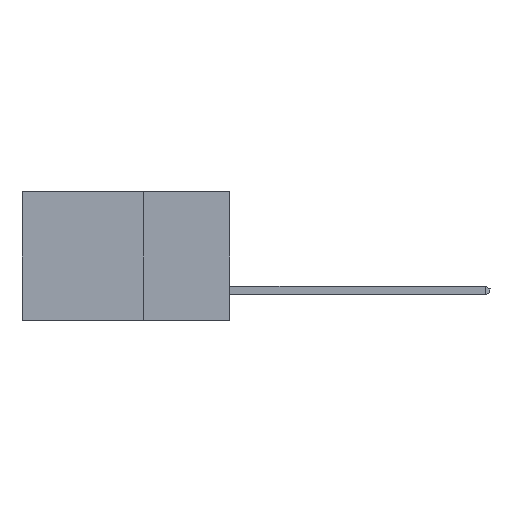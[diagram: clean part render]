
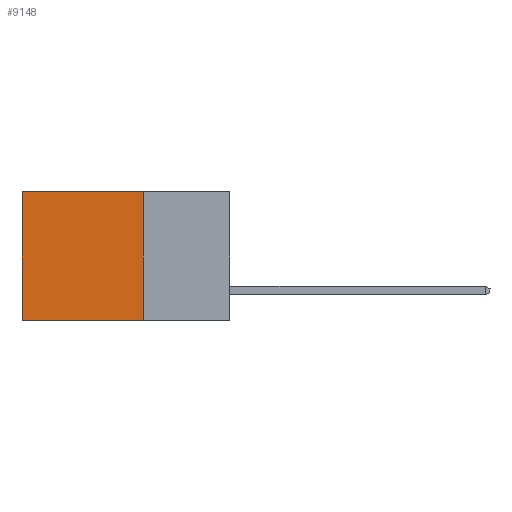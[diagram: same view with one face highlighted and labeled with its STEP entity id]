
A CAD part, left-side view. The second image highlights one B-rep face of the part: STEP entity #9148.
In plain terms, the highlighted planar face has unit normal (-1, 0, 0).
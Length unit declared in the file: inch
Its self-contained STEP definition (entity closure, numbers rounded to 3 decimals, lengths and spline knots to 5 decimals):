
#234 = LINE ( 'NONE', #9749, #6806 ) ;
#680 = ORIENTED_EDGE ( 'NONE', *, *, #12096, .T. ) ;
#724 = LINE ( 'NONE', #6959, #6008 ) ;
#1845 = EDGE_LOOP ( 'NONE', ( #680, #12845, #9667, #8556 ) ) ;
#3047 = VERTEX_POINT ( 'NONE', #14119 ) ;
#3247 = FACE_OUTER_BOUND ( 'NONE', #1845, .T. ) ;
#4720 = CARTESIAN_POINT ( 'NONE',  ( 0.2615, 0.25, -0.37 ) ) ;
#4935 = CARTESIAN_POINT ( 'NONE',  ( 0.2615, 0.6, 0. ) ) ;
#5195 = VERTEX_POINT ( 'NONE', #11747 ) ;
#6008 = VECTOR ( 'NONE', #10463, 39.37008 ) ;
#6310 = DIRECTION ( 'NONE',  ( 0., 0., -1. ) ) ;
#6806 = VECTOR ( 'NONE', #6310, 39.37008 ) ;
#6959 = CARTESIAN_POINT ( 'NONE',  ( 0.2615, 0.25, 0. ) ) ;
#7179 = LINE ( 'NONE', #8269, #8111 ) ;
#7283 = LINE ( 'NONE', #15372, #13956 ) ;
#8012 = DIRECTION ( 'NONE',  ( 1., 0., 0. ) ) ;
#8111 = VECTOR ( 'NONE', #10542, 39.37008 ) ;
#8269 = CARTESIAN_POINT ( 'NONE',  ( 0.2615, 0.6, -0.37 ) ) ;
#8403 = EDGE_CURVE ( 'NONE', #3047, #5195, #234, .T. ) ;
#8556 = ORIENTED_EDGE ( 'NONE', *, *, #13909, .T. ) ;
#8612 = CARTESIAN_POINT ( 'NONE',  ( 0.2615, 0.6, -0.37 ) ) ;
#8659 = EDGE_CURVE ( 'NONE', #5195, #13022, #7283, .T. ) ;
#9148 = ADVANCED_FACE ( 'NONE', ( #3247 ), #15241, .F. ) ;
#9667 = ORIENTED_EDGE ( 'NONE', *, *, #8403, .F. ) ;
#9749 = CARTESIAN_POINT ( 'NONE',  ( 0.2615, 0.25, -0.37 ) ) ;
#10278 = AXIS2_PLACEMENT_3D ( 'NONE', #4720, #8012, #10509 ) ;
#10463 = DIRECTION ( 'NONE',  ( 0., 1., 0. ) ) ;
#10509 = DIRECTION ( 'NONE',  ( 0., 0., -1. ) ) ;
#10542 = DIRECTION ( 'NONE',  ( 0., 0., -1. ) ) ;
#10804 = DIRECTION ( 'NONE',  ( 0., 1., 0. ) ) ;
#10948 = VERTEX_POINT ( 'NONE', #4935 ) ;
#11747 = CARTESIAN_POINT ( 'NONE',  ( 0.2615, 0.25, -0.37 ) ) ;
#12096 = EDGE_CURVE ( 'NONE', #10948, #13022, #7179, .T. ) ;
#12845 = ORIENTED_EDGE ( 'NONE', *, *, #8659, .F. ) ;
#13022 = VERTEX_POINT ( 'NONE', #8612 ) ;
#13909 = EDGE_CURVE ( 'NONE', #3047, #10948, #724, .T. ) ;
#13956 = VECTOR ( 'NONE', #10804, 39.37008 ) ;
#14119 = CARTESIAN_POINT ( 'NONE',  ( 0.2615, 0.25, 0. ) ) ;
#15241 = PLANE ( 'NONE',  #10278 ) ;
#15372 = CARTESIAN_POINT ( 'NONE',  ( 0.2615, 0.25, -0.37 ) ) ;
